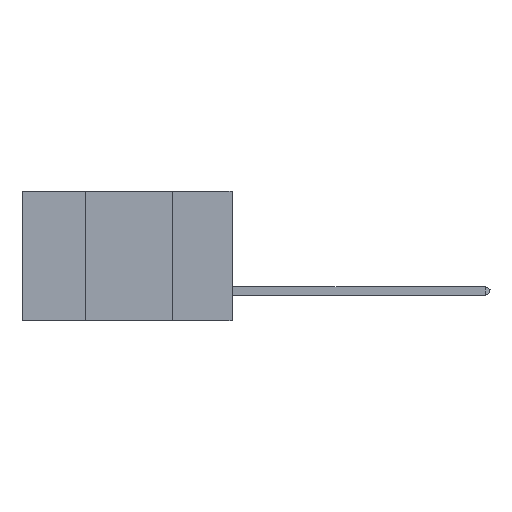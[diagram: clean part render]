
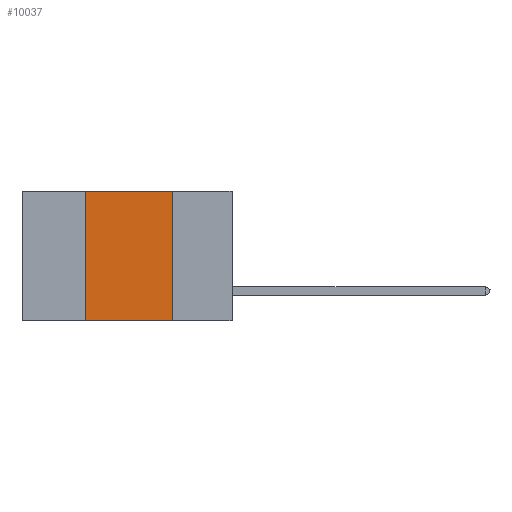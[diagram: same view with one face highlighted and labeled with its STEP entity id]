
A CAD part, left-side view. The second image highlights one B-rep face of the part: STEP entity #10037.
In plain terms, the highlighted planar face has unit normal (-1, 0, 0).
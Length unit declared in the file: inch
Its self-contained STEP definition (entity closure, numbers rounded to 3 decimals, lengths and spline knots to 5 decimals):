
#170 = DIRECTION ( 'NONE',  ( 0., -1., 0. ) ) ;
#702 = CARTESIAN_POINT ( 'NONE',  ( 0., 0.42, 0. ) ) ;
#2842 = CARTESIAN_POINT ( 'NONE',  ( 0., 0.6, 0. ) ) ;
#4094 = VERTEX_POINT ( 'NONE', #28932 ) ;
#6513 = AXIS2_PLACEMENT_3D ( 'NONE', #6667, #21926, #19447 ) ;
#6667 = CARTESIAN_POINT ( 'NONE',  ( 0., 0.6, 0. ) ) ;
#8180 = EDGE_CURVE ( 'NONE', #9564, #17076, #11757, .T. ) ;
#9564 = VERTEX_POINT ( 'NONE', #11745 ) ;
#10037 = ADVANCED_FACE ( 'NONE', ( #16046 ), #21807, .F. ) ;
#10095 = ORIENTED_EDGE ( 'NONE', *, *, #8180, .F. ) ;
#11716 = CARTESIAN_POINT ( 'NONE',  ( 0., 0.42, -0.37 ) ) ;
#11745 = CARTESIAN_POINT ( 'NONE',  ( 0., 0.42, 0. ) ) ;
#11757 = LINE ( 'NONE', #2842, #25614 ) ;
#13008 = LINE ( 'NONE', #27150, #17376 ) ;
#13282 = DIRECTION ( 'NONE',  ( 0., 0., 1. ) ) ;
#15516 = EDGE_LOOP ( 'NONE', ( #16359, #10095, #18522, #15560 ) ) ;
#15560 = ORIENTED_EDGE ( 'NONE', *, *, #20165, .T. ) ;
#16046 = FACE_OUTER_BOUND ( 'NONE', #15516, .T. ) ;
#16359 = ORIENTED_EDGE ( 'NONE', *, *, #27873, .F. ) ;
#17076 = VERTEX_POINT ( 'NONE', #31965 ) ;
#17376 = VECTOR ( 'NONE', #29447, 39.37008 ) ;
#18137 = LINE ( 'NONE', #702, #22156 ) ;
#18296 = CARTESIAN_POINT ( 'NONE',  ( 0., 0.6, -0.37 ) ) ;
#18522 = ORIENTED_EDGE ( 'NONE', *, *, #22985, .F. ) ;
#19447 = DIRECTION ( 'NONE',  ( 0., 0., -1. ) ) ;
#20165 = EDGE_CURVE ( 'NONE', #21166, #4094, #31812, .T. ) ;
#21166 = VERTEX_POINT ( 'NONE', #11716 ) ;
#21807 = PLANE ( 'NONE',  #6513 ) ;
#21926 = DIRECTION ( 'NONE',  ( 1., 0., 0. ) ) ;
#22156 = VECTOR ( 'NONE', #13282, 39.37008 ) ;
#22985 = EDGE_CURVE ( 'NONE', #21166, #9564, #18137, .T. ) ;
#25614 = VECTOR ( 'NONE', #170, 39.37008 ) ;
#25738 = DIRECTION ( 'NONE',  ( 0., -1., 0. ) ) ;
#27150 = CARTESIAN_POINT ( 'NONE',  ( 0., 0.17, 0. ) ) ;
#27873 = EDGE_CURVE ( 'NONE', #17076, #4094, #13008, .T. ) ;
#28624 = VECTOR ( 'NONE', #25738, 39.37008 ) ;
#28932 = CARTESIAN_POINT ( 'NONE',  ( 0., 0.17, -0.37 ) ) ;
#29447 = DIRECTION ( 'NONE',  ( 0., 0., -1. ) ) ;
#31812 = LINE ( 'NONE', #18296, #28624 ) ;
#31965 = CARTESIAN_POINT ( 'NONE',  ( 0., 0.17, 0. ) ) ;
